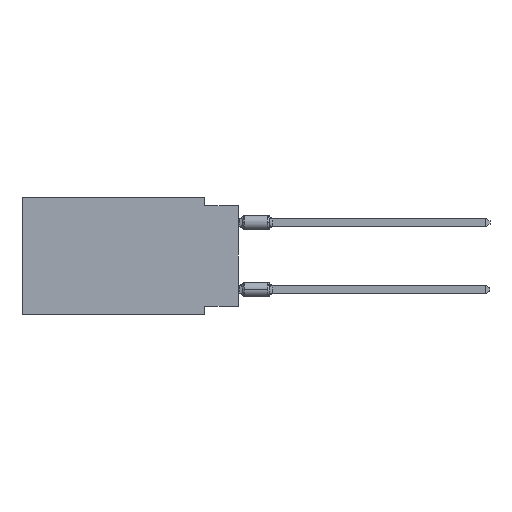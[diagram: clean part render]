
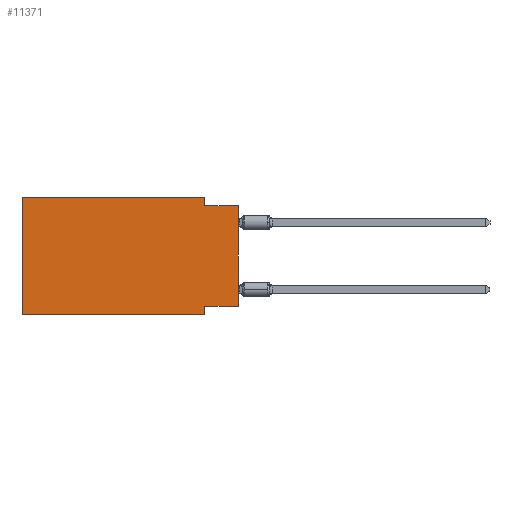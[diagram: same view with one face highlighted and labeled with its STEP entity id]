
A CAD part, left-side view. The second image highlights one B-rep face of the part: STEP entity #11371.
In plain terms, the highlighted planar face has unit normal (-1, 0, 0).
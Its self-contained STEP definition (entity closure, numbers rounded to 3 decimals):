
#762 = DIRECTION ( 'NONE',  ( 0., -1., 0. ) ) ;
#778 = ORIENTED_EDGE ( 'NONE', *, *, #5146, .F. ) ;
#823 = EDGE_CURVE ( 'NONE', #13139, #4666, #19202, .T. ) ;
#912 = DIRECTION ( 'NONE',  ( 0., 0., -1. ) ) ;
#1357 = CARTESIAN_POINT ( 'NONE',  ( 0., 2.54, 0. ) ) ;
#1597 = CARTESIAN_POINT ( 'NONE',  ( 0., 2.54, -8.255 ) ) ;
#1759 = LINE ( 'NONE', #5434, #10055 ) ;
#1942 = DIRECTION ( 'NONE',  ( 0., -1., 0. ) ) ;
#2439 = LINE ( 'NONE', #13855, #19235 ) ;
#2468 = ORIENTED_EDGE ( 'NONE', *, *, #4503, .F. ) ;
#2786 = DIRECTION ( 'NONE',  ( 0., 1., 0. ) ) ;
#3974 = DIRECTION ( 'NONE',  ( 0., -1., 0. ) ) ;
#4349 = LINE ( 'NONE', #17421, #7252 ) ;
#4400 = ORIENTED_EDGE ( 'NONE', *, *, #9492, .T. ) ;
#4503 = EDGE_CURVE ( 'NONE', #10305, #12395, #2439, .T. ) ;
#4627 = CARTESIAN_POINT ( 'NONE',  ( 0., 0., -8.255 ) ) ;
#4666 = VERTEX_POINT ( 'NONE', #12160 ) ;
#5022 = DIRECTION ( 'NONE',  ( 0., 0., 1. ) ) ;
#5146 = EDGE_CURVE ( 'NONE', #10492, #13139, #7341, .T. ) ;
#5434 = CARTESIAN_POINT ( 'NONE',  ( 0., 0., 0. ) ) ;
#6066 = CARTESIAN_POINT ( 'NONE',  ( 0., 16.383, 0. ) ) ;
#6416 = CARTESIAN_POINT ( 'NONE',  ( 0., 2.54, -8.89 ) ) ;
#7115 = DIRECTION ( 'NONE',  ( 0., 0., -1. ) ) ;
#7198 = CARTESIAN_POINT ( 'NONE',  ( 0., 0., -0.635 ) ) ;
#7235 = LINE ( 'NONE', #12256, #15913 ) ;
#7252 = VECTOR ( 'NONE', #762, 1000. ) ;
#7328 = ORIENTED_EDGE ( 'NONE', *, *, #823, .F. ) ;
#7341 = LINE ( 'NONE', #14608, #7721 ) ;
#7501 = EDGE_CURVE ( 'NONE', #16425, #10492, #7235, .T. ) ;
#7721 = VECTOR ( 'NONE', #3974, 1000. ) ;
#7784 = LINE ( 'NONE', #4627, #11545 ) ;
#8247 = ORIENTED_EDGE ( 'NONE', *, *, #7501, .F. ) ;
#9128 = ORIENTED_EDGE ( 'NONE', *, *, #9780, .T. ) ;
#9492 = EDGE_CURVE ( 'NONE', #11892, #10735, #1759, .T. ) ;
#9507 = EDGE_CURVE ( 'NONE', #4666, #10735, #4349, .T. ) ;
#9780 = EDGE_CURVE ( 'NONE', #16425, #12395, #10228, .T. ) ;
#10055 = VECTOR ( 'NONE', #5022, 1000. ) ;
#10228 = LINE ( 'NONE', #12059, #19855 ) ;
#10305 = VERTEX_POINT ( 'NONE', #1597 ) ;
#10492 = VERTEX_POINT ( 'NONE', #11156 ) ;
#10735 = VERTEX_POINT ( 'NONE', #7198 ) ;
#11156 = CARTESIAN_POINT ( 'NONE',  ( 0., 16.383, 0. ) ) ;
#11371 = ADVANCED_FACE ( 'NONE', ( #19688 ), #16189, .F. ) ;
#11545 = VECTOR ( 'NONE', #2786, 1000. ) ;
#11882 = CARTESIAN_POINT ( 'NONE',  ( 0., 16.383, -8.89 ) ) ;
#11892 = VERTEX_POINT ( 'NONE', #16595 ) ;
#12059 = CARTESIAN_POINT ( 'NONE',  ( 0., 16.383, -8.89 ) ) ;
#12160 = CARTESIAN_POINT ( 'NONE',  ( 0., 2.54, -0.635 ) ) ;
#12256 = CARTESIAN_POINT ( 'NONE',  ( 0., 16.383, 0. ) ) ;
#12395 = VERTEX_POINT ( 'NONE', #6416 ) ;
#12493 = VECTOR ( 'NONE', #912, 1000. ) ;
#12736 = EDGE_LOOP ( 'NONE', ( #4400, #19229, #7328, #778, #8247, #9128, #2468, #21411 ) ) ;
#12809 = DIRECTION ( 'NONE',  ( 1., 0., 0. ) ) ;
#13139 = VERTEX_POINT ( 'NONE', #1357 ) ;
#13855 = CARTESIAN_POINT ( 'NONE',  ( 0., 2.54, -8.89 ) ) ;
#14125 = AXIS2_PLACEMENT_3D ( 'NONE', #6066, #12809, #14668 ) ;
#14608 = CARTESIAN_POINT ( 'NONE',  ( 0., 16.383, 0. ) ) ;
#14668 = DIRECTION ( 'NONE',  ( 0., 0., -1. ) ) ;
#15823 = CARTESIAN_POINT ( 'NONE',  ( 0., 2.54, 0. ) ) ;
#15913 = VECTOR ( 'NONE', #16933, 1000. ) ;
#16189 = PLANE ( 'NONE',  #14125 ) ;
#16425 = VERTEX_POINT ( 'NONE', #11882 ) ;
#16595 = CARTESIAN_POINT ( 'NONE',  ( 0., 0., -8.255 ) ) ;
#16933 = DIRECTION ( 'NONE',  ( 0., 0., 1. ) ) ;
#16997 = EDGE_CURVE ( 'NONE', #11892, #10305, #7784, .T. ) ;
#17421 = CARTESIAN_POINT ( 'NONE',  ( 0., 0., -0.635 ) ) ;
#19202 = LINE ( 'NONE', #15823, #12493 ) ;
#19229 = ORIENTED_EDGE ( 'NONE', *, *, #9507, .F. ) ;
#19235 = VECTOR ( 'NONE', #7115, 1000. ) ;
#19688 = FACE_OUTER_BOUND ( 'NONE', #12736, .T. ) ;
#19855 = VECTOR ( 'NONE', #1942, 1000. ) ;
#21411 = ORIENTED_EDGE ( 'NONE', *, *, #16997, .F. ) ;
